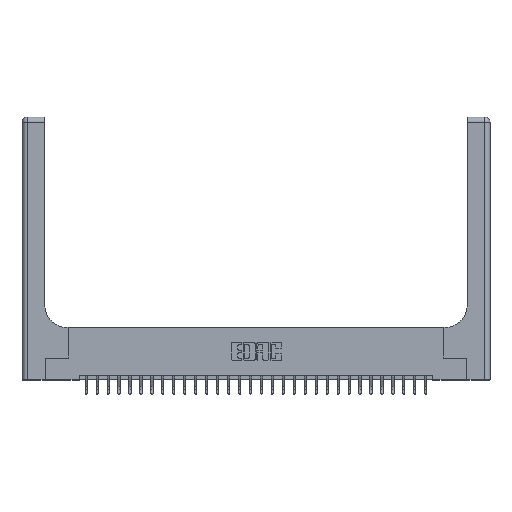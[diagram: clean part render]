
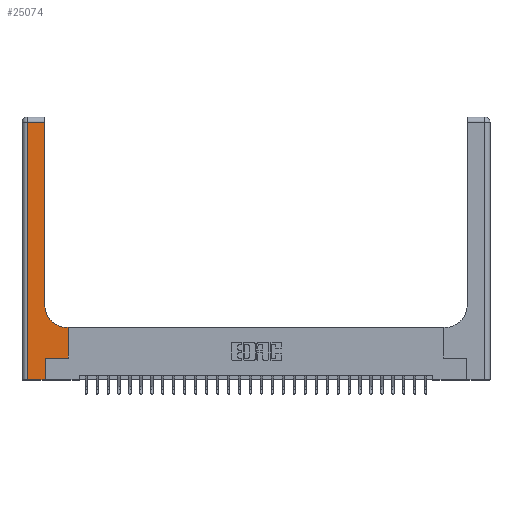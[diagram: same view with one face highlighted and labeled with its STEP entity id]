
A CAD part, top view. The second image highlights one B-rep face of the part: STEP entity #25074.
In plain terms, the highlighted planar face has unit normal (0, 0, 1).
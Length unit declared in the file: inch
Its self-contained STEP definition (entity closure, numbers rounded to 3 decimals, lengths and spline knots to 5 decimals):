
#18 = LINE ( 'NONE', #15266, #25719 ) ;
#19 = VECTOR ( 'NONE', #9687, 39.37008 ) ;
#380 = CARTESIAN_POINT ( 'NONE',  ( 0., 2.94, 0.37 ) ) ;
#440 = ORIENTED_EDGE ( 'NONE', *, *, #7904, .T. ) ;
#1816 = FACE_OUTER_BOUND ( 'NONE', #11034, .T. ) ;
#1880 = CARTESIAN_POINT ( 'NONE',  ( 0., 0., 0.37 ) ) ;
#2009 = ORIENTED_EDGE ( 'NONE', *, *, #16702, .T. ) ;
#2924 = VERTEX_POINT ( 'NONE', #27770 ) ;
#3149 = ORIENTED_EDGE ( 'NONE', *, *, #22568, .T. ) ;
#3517 = ORIENTED_EDGE ( 'NONE', *, *, #7083, .T. ) ;
#3740 = LINE ( 'NONE', #1880, #16826 ) ;
#4953 = AXIS2_PLACEMENT_3D ( 'NONE', #19187, #20894, #16512 ) ;
#5078 = EDGE_CURVE ( 'NONE', #17191, #6938, #26132, .T. ) ;
#5202 = CARTESIAN_POINT ( 'NONE',  ( 0.06, 2.94, 0.37 ) ) ;
#6938 = VERTEX_POINT ( 'NONE', #5202 ) ;
#7083 = EDGE_CURVE ( 'NONE', #14413, #2924, #13843, .T. ) ;
#7633 = EDGE_CURVE ( 'NONE', #13683, #12002, #8685, .T. ) ;
#7686 = DIRECTION ( 'NONE',  ( -1., 0., 0. ) ) ;
#7904 = EDGE_CURVE ( 'NONE', #6938, #18518, #25197, .T. ) ;
#8685 = CIRCLE ( 'NONE', #17776, 0.25 ) ;
#8899 = VERTEX_POINT ( 'NONE', #15587 ) ;
#8948 = VECTOR ( 'NONE', #7686, 39.37008 ) ;
#9277 = LINE ( 'NONE', #15700, #11137 ) ;
#9687 = DIRECTION ( 'NONE',  ( 0., 1., 0. ) ) ;
#10419 = DIRECTION ( 'NONE',  ( 0., -1., 0. ) ) ;
#10589 = EDGE_CURVE ( 'NONE', #18518, #8899, #3740, .T. ) ;
#10778 = CARTESIAN_POINT ( 'NONE',  ( 0.26, 3., 0.37 ) ) ;
#11034 = EDGE_LOOP ( 'NONE', ( #26329, #19701, #440, #27631, #15762, #2009, #3517, #3149, #25709 ) ) ;
#11137 = VECTOR ( 'NONE', #11423, 39.37008 ) ;
#11423 = DIRECTION ( 'NONE',  ( 1., 0., 0. ) ) ;
#12002 = VERTEX_POINT ( 'NONE', #12131 ) ;
#12131 = CARTESIAN_POINT ( 'NONE',  ( 0.26, 0.85, 0.37 ) ) ;
#12803 = CARTESIAN_POINT ( 'NONE',  ( 0.265, 0.25, 0.37 ) ) ;
#13683 = VERTEX_POINT ( 'NONE', #24858 ) ;
#13843 = LINE ( 'NONE', #27014, #19 ) ;
#13856 = VECTOR ( 'NONE', #14178, 39.37008 ) ;
#14178 = DIRECTION ( 'NONE',  ( -1., 0., 0. ) ) ;
#14220 = DIRECTION ( 'NONE',  ( 0., 0., -1. ) ) ;
#14413 = VERTEX_POINT ( 'NONE', #24092 ) ;
#15133 = VERTEX_POINT ( 'NONE', #12803 ) ;
#15266 = CARTESIAN_POINT ( 'NONE',  ( 0.265, 0., 0.37 ) ) ;
#15488 = LINE ( 'NONE', #10778, #27883 ) ;
#15545 = VECTOR ( 'NONE', #10419, 39.37008 ) ;
#15587 = CARTESIAN_POINT ( 'NONE',  ( 0.265, 0., 0.37 ) ) ;
#15700 = CARTESIAN_POINT ( 'NONE',  ( 0.265, 0.25, 0.37 ) ) ;
#15725 = EDGE_CURVE ( 'NONE', #12002, #17191, #15488, .T. ) ;
#15762 = ORIENTED_EDGE ( 'NONE', *, *, #22427, .T. ) ;
#15969 = CARTESIAN_POINT ( 'NONE',  ( 0.26, 0.6, 0.37 ) ) ;
#16081 = CARTESIAN_POINT ( 'NONE',  ( 0.06, 0., 0.37 ) ) ;
#16512 = DIRECTION ( 'NONE',  ( -1., 0., 0. ) ) ;
#16702 = EDGE_CURVE ( 'NONE', #15133, #14413, #9277, .T. ) ;
#16826 = VECTOR ( 'NONE', #27889, 39.37008 ) ;
#17191 = VERTEX_POINT ( 'NONE', #22151 ) ;
#17324 = DIRECTION ( 'NONE',  ( 0., 1., 0. ) ) ;
#17776 = AXIS2_PLACEMENT_3D ( 'NONE', #24976, #14220, #22823 ) ;
#18518 = VERTEX_POINT ( 'NONE', #16081 ) ;
#19187 = CARTESIAN_POINT ( 'NONE',  ( 0., 3., 0.37 ) ) ;
#19701 = ORIENTED_EDGE ( 'NONE', *, *, #5078, .T. ) ;
#20894 = DIRECTION ( 'NONE',  ( 0., 0., -1. ) ) ;
#22151 = CARTESIAN_POINT ( 'NONE',  ( 0.26, 2.94, 0.37 ) ) ;
#22427 = EDGE_CURVE ( 'NONE', #8899, #15133, #18, .T. ) ;
#22568 = EDGE_CURVE ( 'NONE', #2924, #13683, #27161, .T. ) ;
#22823 = DIRECTION ( 'NONE',  ( 1., 0., 0. ) ) ;
#23561 = PLANE ( 'NONE',  #4953 ) ;
#24092 = CARTESIAN_POINT ( 'NONE',  ( 0.528, 0.25, 0.37 ) ) ;
#24858 = CARTESIAN_POINT ( 'NONE',  ( 0.51, 0.6, 0.37 ) ) ;
#24976 = CARTESIAN_POINT ( 'NONE',  ( 0.51, 0.85, 0.37 ) ) ;
#25074 = ADVANCED_FACE ( 'NONE', ( #1816 ), #23561, .F. ) ;
#25197 = LINE ( 'NONE', #25329, #15545 ) ;
#25329 = CARTESIAN_POINT ( 'NONE',  ( 0.06, 3., 0.37 ) ) ;
#25709 = ORIENTED_EDGE ( 'NONE', *, *, #7633, .T. ) ;
#25719 = VECTOR ( 'NONE', #26321, 39.37008 ) ;
#26132 = LINE ( 'NONE', #380, #13856 ) ;
#26321 = DIRECTION ( 'NONE',  ( 0., 1., 0. ) ) ;
#26329 = ORIENTED_EDGE ( 'NONE', *, *, #15725, .T. ) ;
#27014 = CARTESIAN_POINT ( 'NONE',  ( 0.528, 0.25, 0.37 ) ) ;
#27161 = LINE ( 'NONE', #15969, #8948 ) ;
#27631 = ORIENTED_EDGE ( 'NONE', *, *, #10589, .T. ) ;
#27770 = CARTESIAN_POINT ( 'NONE',  ( 0.528, 0.6, 0.37 ) ) ;
#27883 = VECTOR ( 'NONE', #17324, 39.37008 ) ;
#27889 = DIRECTION ( 'NONE',  ( 1., 0., 0. ) ) ;
